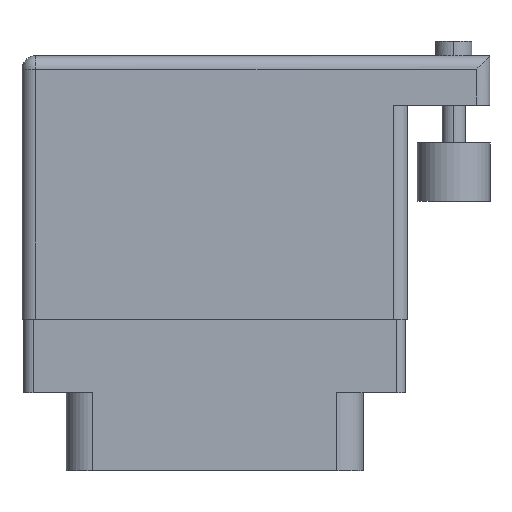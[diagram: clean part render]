
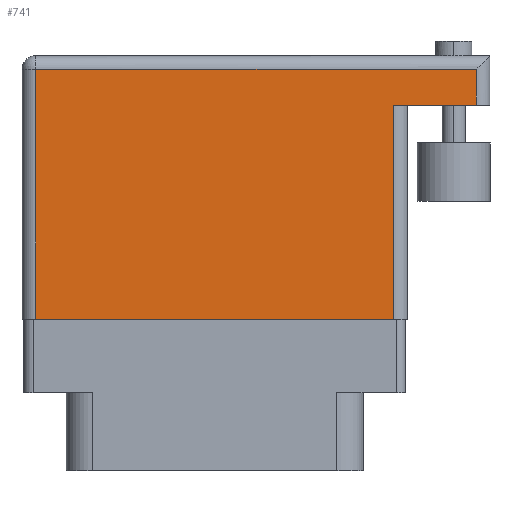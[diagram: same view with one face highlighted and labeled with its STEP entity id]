
A CAD part, front view. The second image highlights one B-rep face of the part: STEP entity #741.
In plain terms, the highlighted face is planar.
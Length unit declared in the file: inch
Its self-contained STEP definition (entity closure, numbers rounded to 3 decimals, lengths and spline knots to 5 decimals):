
#74 = VECTOR ( 'NONE', #3499, 39.37008 ) ;
#374 = CARTESIAN_POINT ( 'NONE',  ( 0.047, 0., 0. ) ) ;
#623 = EDGE_CURVE ( 'NONE', #20465, #740, #5927, .T. ) ;
#740 = VERTEX_POINT ( 'NONE', #2248 ) ;
#741 = ADVANCED_FACE ( 'NONE', ( #7003 ), #20891, .F. ) ;
#1024 = EDGE_CURVE ( 'NONE', #17962, #19083, #13670, .T. ) ;
#1073 = ORIENTED_EDGE ( 'NONE', *, *, #11206, .T. ) ;
#2015 = ORIENTED_EDGE ( 'NONE', *, *, #14831, .T. ) ;
#2171 = ORIENTED_EDGE ( 'NONE', *, *, #623, .T. ) ;
#2248 = CARTESIAN_POINT ( 'NONE',  ( 1.562, 0.859, 0. ) ) ;
#2659 = VECTOR ( 'NONE', #11297, 39.37008 ) ;
#2797 = DIRECTION ( 'NONE',  ( 0., 1., 0. ) ) ;
#3112 = CARTESIAN_POINT ( 'NONE',  ( 0.047, 0., 0. ) ) ;
#3457 = CARTESIAN_POINT ( 'NONE',  ( 1.562, 0.736, 0. ) ) ;
#3499 = DIRECTION ( 'NONE',  ( 1., 0., 0. ) ) ;
#3926 = DIRECTION ( 'NONE',  ( 0., -1., 0. ) ) ;
#4584 = VECTOR ( 'NONE', #12487, 39.37008 ) ;
#4875 = EDGE_CURVE ( 'NONE', #12733, #17962, #13498, .T. ) ;
#5912 = CARTESIAN_POINT ( 'NONE',  ( 0., 0.859, 0. ) ) ;
#5927 = LINE ( 'NONE', #10404, #11302 ) ;
#6781 = CARTESIAN_POINT ( 'NONE',  ( 0., 0., 0. ) ) ;
#6796 = CARTESIAN_POINT ( 'NONE',  ( 1.278, 0., 0. ) ) ;
#7000 = ORIENTED_EDGE ( 'NONE', *, *, #1024, .T. ) ;
#7003 = FACE_OUTER_BOUND ( 'NONE', #20393, .T. ) ;
#8831 = CARTESIAN_POINT ( 'NONE',  ( 0.047, 0.859, 0. ) ) ;
#9279 = LINE ( 'NONE', #11239, #20440 ) ;
#10404 = CARTESIAN_POINT ( 'NONE',  ( 1.562, 0.906, 0. ) ) ;
#10634 = EDGE_CURVE ( 'NONE', #20465, #21333, #12012, .T. ) ;
#10721 = LINE ( 'NONE', #5912, #4584 ) ;
#10983 = CARTESIAN_POINT ( 'NONE',  ( 0., 0.906, 0. ) ) ;
#11206 = EDGE_CURVE ( 'NONE', #19083, #21333, #9279, .T. ) ;
#11239 = CARTESIAN_POINT ( 'NONE',  ( 1.278, 0.736, 0. ) ) ;
#11297 = DIRECTION ( 'NONE',  ( -1., 0., 0. ) ) ;
#11302 = VECTOR ( 'NONE', #17433, 39.37008 ) ;
#12012 = LINE ( 'NONE', #16438, #2659 ) ;
#12451 = AXIS2_PLACEMENT_3D ( 'NONE', #10983, #12684, #17809 ) ;
#12487 = DIRECTION ( 'NONE',  ( -1., 0., 0. ) ) ;
#12684 = DIRECTION ( 'NONE',  ( 0., 0., -1. ) ) ;
#12733 = VERTEX_POINT ( 'NONE', #8831 ) ;
#13498 = LINE ( 'NONE', #374, #16949 ) ;
#13670 = LINE ( 'NONE', #6781, #74 ) ;
#13897 = ORIENTED_EDGE ( 'NONE', *, *, #4875, .T. ) ;
#14831 = EDGE_CURVE ( 'NONE', #740, #12733, #10721, .T. ) ;
#15340 = CARTESIAN_POINT ( 'NONE',  ( 1.278, 0.736, 0. ) ) ;
#15927 = ORIENTED_EDGE ( 'NONE', *, *, #10634, .F. ) ;
#16438 = CARTESIAN_POINT ( 'NONE',  ( 1.609, 0.736, 0. ) ) ;
#16949 = VECTOR ( 'NONE', #3926, 39.37008 ) ;
#17433 = DIRECTION ( 'NONE',  ( 0., 1., 0. ) ) ;
#17809 = DIRECTION ( 'NONE',  ( -1., 0., 0. ) ) ;
#17962 = VERTEX_POINT ( 'NONE', #3112 ) ;
#19083 = VERTEX_POINT ( 'NONE', #6796 ) ;
#20393 = EDGE_LOOP ( 'NONE', ( #7000, #1073, #15927, #2171, #2015, #13897 ) ) ;
#20440 = VECTOR ( 'NONE', #2797, 39.37008 ) ;
#20465 = VERTEX_POINT ( 'NONE', #3457 ) ;
#20891 = PLANE ( 'NONE',  #12451 ) ;
#21333 = VERTEX_POINT ( 'NONE', #15340 ) ;
